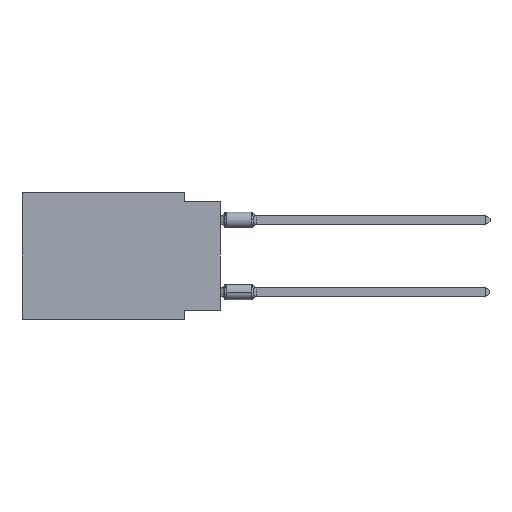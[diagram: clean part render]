
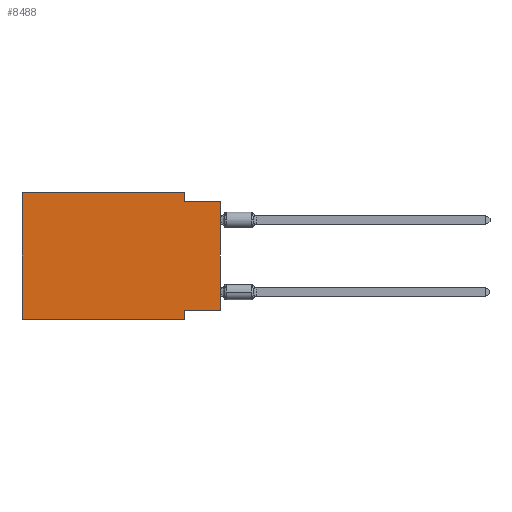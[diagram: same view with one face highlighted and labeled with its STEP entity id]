
A CAD part, left-side view. The second image highlights one B-rep face of the part: STEP entity #8488.
In plain terms, the highlighted planar face has unit normal (-1, 0, 0).
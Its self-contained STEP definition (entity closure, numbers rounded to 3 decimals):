
#98 = LINE ( 'NONE', #9696, #5197 ) ;
#236 = LINE ( 'NONE', #2489, #6669 ) ;
#606 = EDGE_CURVE ( 'NONE', #14377, #6790, #5737, .T. ) ;
#625 = EDGE_CURVE ( 'NONE', #14835, #11110, #15007, .T. ) ;
#635 = CARTESIAN_POINT ( 'NONE',  ( 0., 2.54, -8.255 ) ) ;
#1153 = CARTESIAN_POINT ( 'NONE',  ( 0., 2.54, 0. ) ) ;
#1237 = DIRECTION ( 'NONE',  ( 1., 0., 0. ) ) ;
#1297 = EDGE_CURVE ( 'NONE', #8384, #10764, #3497, .T. ) ;
#2005 = LINE ( 'NONE', #6693, #13829 ) ;
#2396 = DIRECTION ( 'NONE',  ( 0., 0., -1. ) ) ;
#2474 = PLANE ( 'NONE',  #10649 ) ;
#2481 = VECTOR ( 'NONE', #10511, 1000. ) ;
#2489 = CARTESIAN_POINT ( 'NONE',  ( 0., 0., -0.635 ) ) ;
#3372 = VECTOR ( 'NONE', #12618, 1000. ) ;
#3465 = EDGE_CURVE ( 'NONE', #11110, #9843, #6997, .T. ) ;
#3497 = LINE ( 'NONE', #12614, #10758 ) ;
#3641 = ORIENTED_EDGE ( 'NONE', *, *, #1297, .T. ) ;
#3709 = CARTESIAN_POINT ( 'NONE',  ( 0., 2.54, -8.89 ) ) ;
#3713 = DIRECTION ( 'NONE',  ( 0., 1., 0. ) ) ;
#3877 = VECTOR ( 'NONE', #11962, 1000. ) ;
#4224 = EDGE_CURVE ( 'NONE', #9843, #10764, #236, .T. ) ;
#4658 = CARTESIAN_POINT ( 'NONE',  ( 0., 2.54, 0. ) ) ;
#5197 = VECTOR ( 'NONE', #3713, 1000. ) ;
#5285 = CARTESIAN_POINT ( 'NONE',  ( 0., 0., -0.635 ) ) ;
#5737 = LINE ( 'NONE', #10251, #3372 ) ;
#6216 = ORIENTED_EDGE ( 'NONE', *, *, #625, .F. ) ;
#6669 = VECTOR ( 'NONE', #9619, 1000. ) ;
#6693 = CARTESIAN_POINT ( 'NONE',  ( 0., 13.97, 0. ) ) ;
#6790 = VERTEX_POINT ( 'NONE', #3709 ) ;
#6997 = LINE ( 'NONE', #1153, #2481 ) ;
#7299 = FACE_OUTER_BOUND ( 'NONE', #9590, .T. ) ;
#7347 = ORIENTED_EDGE ( 'NONE', *, *, #606, .F. ) ;
#7889 = ORIENTED_EDGE ( 'NONE', *, *, #14922, .F. ) ;
#8034 = DIRECTION ( 'NONE',  ( 0., 0., 1. ) ) ;
#8368 = ORIENTED_EDGE ( 'NONE', *, *, #3465, .F. ) ;
#8384 = VERTEX_POINT ( 'NONE', #13616 ) ;
#8488 = ADVANCED_FACE ( 'NONE', ( #7299 ), #2474, .F. ) ;
#9590 = EDGE_LOOP ( 'NONE', ( #3641, #11824, #8368, #6216, #7889, #12756, #7347, #13992 ) ) ;
#9603 = LINE ( 'NONE', #14278, #3877 ) ;
#9619 = DIRECTION ( 'NONE',  ( 0., -1., 0. ) ) ;
#9696 = CARTESIAN_POINT ( 'NONE',  ( 0., 0., -8.255 ) ) ;
#9843 = VERTEX_POINT ( 'NONE', #13004 ) ;
#10251 = CARTESIAN_POINT ( 'NONE',  ( 0., 2.54, -8.89 ) ) ;
#10300 = EDGE_CURVE ( 'NONE', #14077, #6790, #9603, .T. ) ;
#10401 = DIRECTION ( 'NONE',  ( 0., -1., 0. ) ) ;
#10511 = DIRECTION ( 'NONE',  ( 0., 0., -1. ) ) ;
#10649 = AXIS2_PLACEMENT_3D ( 'NONE', #10806, #1237, #2396 ) ;
#10758 = VECTOR ( 'NONE', #8034, 1000. ) ;
#10764 = VERTEX_POINT ( 'NONE', #5285 ) ;
#10806 = CARTESIAN_POINT ( 'NONE',  ( 0., 13.97, 0. ) ) ;
#11110 = VERTEX_POINT ( 'NONE', #4658 ) ;
#11432 = DIRECTION ( 'NONE',  ( 0., 0., 1. ) ) ;
#11824 = ORIENTED_EDGE ( 'NONE', *, *, #4224, .F. ) ;
#11962 = DIRECTION ( 'NONE',  ( 0., -1., 0. ) ) ;
#12177 = VECTOR ( 'NONE', #10401, 1000. ) ;
#12420 = CARTESIAN_POINT ( 'NONE',  ( 0., 13.97, 0. ) ) ;
#12614 = CARTESIAN_POINT ( 'NONE',  ( 0., 0., 0. ) ) ;
#12618 = DIRECTION ( 'NONE',  ( 0., 0., -1. ) ) ;
#12756 = ORIENTED_EDGE ( 'NONE', *, *, #10300, .T. ) ;
#13004 = CARTESIAN_POINT ( 'NONE',  ( 0., 2.54, -0.635 ) ) ;
#13011 = EDGE_CURVE ( 'NONE', #8384, #14377, #98, .T. ) ;
#13616 = CARTESIAN_POINT ( 'NONE',  ( 0., 0., -8.255 ) ) ;
#13829 = VECTOR ( 'NONE', #11432, 1000. ) ;
#13928 = CARTESIAN_POINT ( 'NONE',  ( 0., 13.97, 0. ) ) ;
#13992 = ORIENTED_EDGE ( 'NONE', *, *, #13011, .F. ) ;
#14077 = VERTEX_POINT ( 'NONE', #14081 ) ;
#14081 = CARTESIAN_POINT ( 'NONE',  ( 0., 13.97, -8.89 ) ) ;
#14278 = CARTESIAN_POINT ( 'NONE',  ( 0., 13.97, -8.89 ) ) ;
#14377 = VERTEX_POINT ( 'NONE', #635 ) ;
#14835 = VERTEX_POINT ( 'NONE', #12420 ) ;
#14922 = EDGE_CURVE ( 'NONE', #14077, #14835, #2005, .T. ) ;
#15007 = LINE ( 'NONE', #13928, #12177 ) ;
